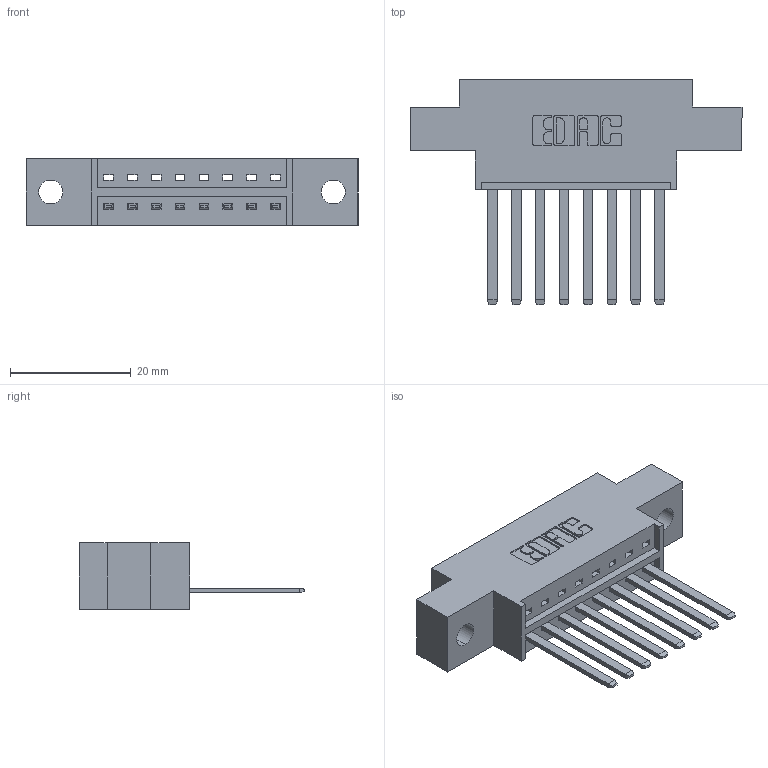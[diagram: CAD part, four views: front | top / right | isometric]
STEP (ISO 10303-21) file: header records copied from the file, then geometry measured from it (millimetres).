
FILE_DESCRIPTION (( 'STEP AP203' ), '1' );
FILE_NAME ('336-008-541-604.STEP', '2020-08-07T19:21:33', ( '' ), ( '' ), 'SwSTEP 2.0', 'SolidWorks 2020', '' );
FILE_SCHEMA (( 'CONFIG_CONTROL_DESIGN' ));
Length unit declared in the file: inch
Products named in the file (3): 336-008-541-604; 336 Part_Offset - .156 Dia - TH; 336-290-001_336-290-541
Assembly tree (9 placements, depth 2):
  336-008-541-604
    336 Part_Offset - .156 Dia - TH
    336-290-001_336-290-541  x8
Bounding box: 55.09 x 37.34 x 11.1 mm (x, y, z)
Volume: 6956.2 mm3; surface area: 7017.1 mm2
Topology: 9 solids, 9 shells, 518 faces, 1555 edges, 1030 vertices
Faces by surface type: plane 346, cylinder 172
Entity records: 10198 total; most frequent: CARTESIAN_POINT 1865, ORIENTED_EDGE 1710, DIRECTION 1543, EDGE_CURVE 855, LINE 723, VECTOR 723, VERTEX_POINT 568, AXIS2_PLACEMENT_3D 410
